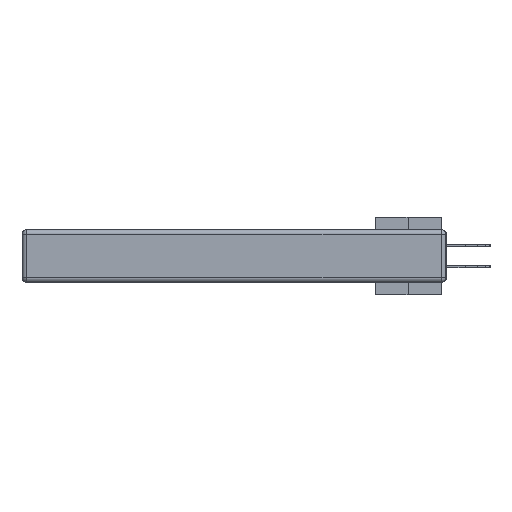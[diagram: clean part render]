
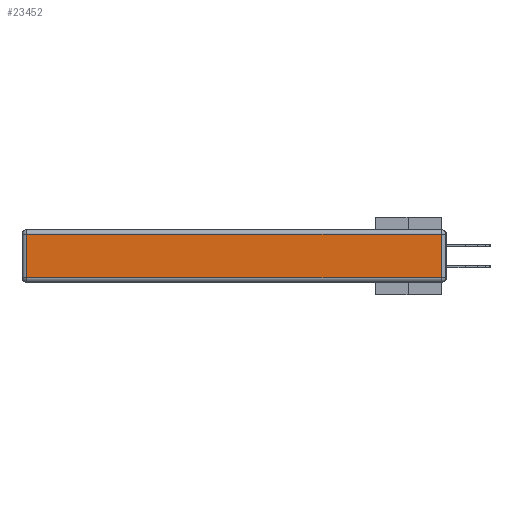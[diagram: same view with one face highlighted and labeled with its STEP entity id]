
A CAD part, left-side view. The second image highlights one B-rep face of the part: STEP entity #23452.
In plain terms, the highlighted planar face has unit normal (-1, 0, 0).
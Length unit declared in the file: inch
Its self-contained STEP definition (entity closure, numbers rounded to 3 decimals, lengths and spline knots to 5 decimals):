
#605 = AXIS2_PLACEMENT_3D ( 'NONE', #20310, #13442, #36387 ) ;
#1194 = ORIENTED_EDGE ( 'NONE', *, *, #19643, .T. ) ;
#1687 = VERTEX_POINT ( 'NONE', #40691 ) ;
#5113 = EDGE_CURVE ( 'NONE', #21507, #17114, #16221, .T. ) ;
#7458 = VERTEX_POINT ( 'NONE', #24747 ) ;
#8508 = VECTOR ( 'NONE', #34308, 39.37008 ) ;
#9962 = DIRECTION ( 'NONE',  ( 0., 0., 1. ) ) ;
#10054 = CARTESIAN_POINT ( 'NONE',  ( 0., 2.72, -0.03 ) ) ;
#13297 = PLANE ( 'NONE',  #605 ) ;
#13365 = LINE ( 'NONE', #26595, #23604 ) ;
#13442 = DIRECTION ( 'NONE',  ( -1., 0., 0. ) ) ;
#14213 = LINE ( 'NONE', #26651, #18748 ) ;
#14620 = EDGE_CURVE ( 'NONE', #17114, #1687, #14213, .T. ) ;
#15629 = CARTESIAN_POINT ( 'NONE',  ( 0., 2.75, -0.03 ) ) ;
#16221 = LINE ( 'NONE', #17427, #8508 ) ;
#17114 = VERTEX_POINT ( 'NONE', #30133 ) ;
#17427 = CARTESIAN_POINT ( 'NONE',  ( 0., 2.72, -0.343 ) ) ;
#18748 = VECTOR ( 'NONE', #29908, 39.37008 ) ;
#19643 = EDGE_CURVE ( 'NONE', #1687, #7458, #13365, .T. ) ;
#20310 = CARTESIAN_POINT ( 'NONE',  ( 0., 0., -0.343 ) ) ;
#20947 = LINE ( 'NONE', #15629, #26069 ) ;
#21004 = EDGE_CURVE ( 'NONE', #7458, #21507, #20947, .T. ) ;
#21507 = VERTEX_POINT ( 'NONE', #10054 ) ;
#22726 = ORIENTED_EDGE ( 'NONE', *, *, #21004, .T. ) ;
#23452 = ADVANCED_FACE ( 'NONE', ( #31658 ), #13297, .T. ) ;
#23604 = VECTOR ( 'NONE', #9962, 39.37008 ) ;
#24142 = ORIENTED_EDGE ( 'NONE', *, *, #14620, .T. ) ;
#24747 = CARTESIAN_POINT ( 'NONE',  ( 0., 0.03, -0.03 ) ) ;
#25214 = DIRECTION ( 'NONE',  ( 0., 1., 0. ) ) ;
#26069 = VECTOR ( 'NONE', #25214, 39.37008 ) ;
#26595 = CARTESIAN_POINT ( 'NONE',  ( 0., 0.03, -0.343 ) ) ;
#26651 = CARTESIAN_POINT ( 'NONE',  ( 0., 0., -0.313 ) ) ;
#29908 = DIRECTION ( 'NONE',  ( 0., -1., 0. ) ) ;
#30133 = CARTESIAN_POINT ( 'NONE',  ( 0., 2.72, -0.313 ) ) ;
#31658 = FACE_OUTER_BOUND ( 'NONE', #34292, .T. ) ;
#34292 = EDGE_LOOP ( 'NONE', ( #24142, #1194, #22726, #37997 ) ) ;
#34308 = DIRECTION ( 'NONE',  ( 0., 0., -1. ) ) ;
#36387 = DIRECTION ( 'NONE',  ( 0., 0., 1. ) ) ;
#37997 = ORIENTED_EDGE ( 'NONE', *, *, #5113, .T. ) ;
#40691 = CARTESIAN_POINT ( 'NONE',  ( 0., 0.03, -0.313 ) ) ;
